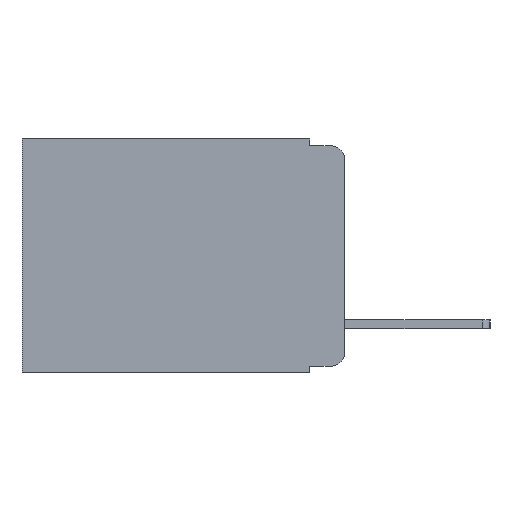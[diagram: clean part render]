
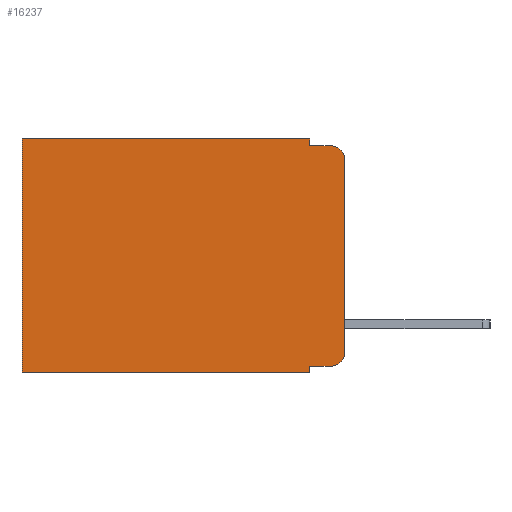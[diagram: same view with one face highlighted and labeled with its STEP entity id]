
A CAD part, left-side view. The second image highlights one B-rep face of the part: STEP entity #16237.
In plain terms, the highlighted planar face has unit normal (-1, 0, 0).
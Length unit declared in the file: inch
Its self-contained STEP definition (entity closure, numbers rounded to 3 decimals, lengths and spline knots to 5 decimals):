
#30 = ORIENTED_EDGE ( 'NONE', *, *, #7770, .T. ) ;
#162 = DIRECTION ( 'NONE',  ( 0., 0., -1. ) ) ;
#414 = ORIENTED_EDGE ( 'NONE', *, *, #9971, .T. ) ;
#877 = VERTEX_POINT ( 'NONE', #4675 ) ;
#891 = CARTESIAN_POINT ( 'NONE',  ( 0.298, 0.051, 0. ) ) ;
#1987 = CARTESIAN_POINT ( 'NONE',  ( 0.298, 0.02, -0.01 ) ) ;
#2524 = VECTOR ( 'NONE', #8147, 39.37008 ) ;
#2715 = VERTEX_POINT ( 'NONE', #1987 ) ;
#3060 = VECTOR ( 'NONE', #19576, 39.37008 ) ;
#3420 = AXIS2_PLACEMENT_3D ( 'NONE', #16864, #5910, #18692 ) ;
#3808 = EDGE_CURVE ( 'NONE', #14345, #7878, #23529, .T. ) ;
#4283 = CARTESIAN_POINT ( 'NONE',  ( 0.298, 0.473, -0.343 ) ) ;
#4372 = CARTESIAN_POINT ( 'NONE',  ( 0.298, 0.02, -0.313 ) ) ;
#4472 = EDGE_CURVE ( 'NONE', #6356, #877, #17974, .T. ) ;
#4675 = CARTESIAN_POINT ( 'NONE',  ( 0.298, 0.051, -0.01 ) ) ;
#5412 = VERTEX_POINT ( 'NONE', #4283 ) ;
#5910 = DIRECTION ( 'NONE',  ( -1., 0., 0. ) ) ;
#6225 = VECTOR ( 'NONE', #12115, 39.37008 ) ;
#6262 = CARTESIAN_POINT ( 'NONE',  ( 0.298, 0., -0.313 ) ) ;
#6305 = DIRECTION ( 'NONE',  ( 0., 0., -1. ) ) ;
#6356 = VERTEX_POINT ( 'NONE', #14288 ) ;
#6496 = VERTEX_POINT ( 'NONE', #21785 ) ;
#7347 = VECTOR ( 'NONE', #19860, 39.37008 ) ;
#7444 = ORIENTED_EDGE ( 'NONE', *, *, #21544, .F. ) ;
#7580 = LINE ( 'NONE', #13575, #2524 ) ;
#7753 = PLANE ( 'NONE',  #16686 ) ;
#7770 = EDGE_CURVE ( 'NONE', #14345, #2715, #19234, .T. ) ;
#7878 = VERTEX_POINT ( 'NONE', #6262 ) ;
#8122 = ORIENTED_EDGE ( 'NONE', *, *, #12481, .T. ) ;
#8147 = DIRECTION ( 'NONE',  ( 0., -1., 0. ) ) ;
#8908 = VECTOR ( 'NONE', #19803, 39.37008 ) ;
#9217 = VECTOR ( 'NONE', #9309, 39.37008 ) ;
#9309 = DIRECTION ( 'NONE',  ( 0., 0., -1. ) ) ;
#9953 = CARTESIAN_POINT ( 'NONE',  ( 0.298, 0.051, -0.01 ) ) ;
#9971 = EDGE_CURVE ( 'NONE', #12214, #7878, #18756, .T. ) ;
#10172 = AXIS2_PLACEMENT_3D ( 'NONE', #4372, #17206, #6305 ) ;
#10758 = ORIENTED_EDGE ( 'NONE', *, *, #3808, .F. ) ;
#11193 = DIRECTION ( 'NONE',  ( 0., 0., -1. ) ) ;
#11417 = DIRECTION ( 'NONE',  ( 1., 0., 0. ) ) ;
#11802 = DIRECTION ( 'NONE',  ( 0., -1., 0. ) ) ;
#12115 = DIRECTION ( 'NONE',  ( 0., 0., -1. ) ) ;
#12214 = VERTEX_POINT ( 'NONE', #21737 ) ;
#12231 = FACE_OUTER_BOUND ( 'NONE', #12458, .T. ) ;
#12458 = EDGE_LOOP ( 'NONE', ( #10758, #30, #15771, #22301, #12653, #18319, #7444, #18349, #8122, #414 ) ) ;
#12481 = EDGE_CURVE ( 'NONE', #18225, #12214, #7580, .T. ) ;
#12653 = ORIENTED_EDGE ( 'NONE', *, *, #16682, .T. ) ;
#13575 = CARTESIAN_POINT ( 'NONE',  ( 0.298, 0.051, -0.333 ) ) ;
#14161 = CARTESIAN_POINT ( 'NONE',  ( 0.298, 0., -0.343 ) ) ;
#14288 = CARTESIAN_POINT ( 'NONE',  ( 0.298, 0.051, 0. ) ) ;
#14345 = VERTEX_POINT ( 'NONE', #15880 ) ;
#14607 = EDGE_CURVE ( 'NONE', #6496, #5412, #22913, .T. ) ;
#14726 = CARTESIAN_POINT ( 'NONE',  ( 0.298, 0., 0. ) ) ;
#15369 = CARTESIAN_POINT ( 'NONE',  ( 0.298, 0.051, -0.333 ) ) ;
#15426 = EDGE_CURVE ( 'NONE', #18225, #16553, #20183, .T. ) ;
#15526 = VECTOR ( 'NONE', #11802, 39.37008 ) ;
#15771 = ORIENTED_EDGE ( 'NONE', *, *, #18252, .F. ) ;
#15880 = CARTESIAN_POINT ( 'NONE',  ( 0.298, 0., -0.03 ) ) ;
#16237 = ADVANCED_FACE ( 'NONE', ( #12231 ), #7753, .F. ) ;
#16553 = VERTEX_POINT ( 'NONE', #17736 ) ;
#16682 = EDGE_CURVE ( 'NONE', #6356, #6496, #22306, .T. ) ;
#16686 = AXIS2_PLACEMENT_3D ( 'NONE', #22183, #11417, #162 ) ;
#16864 = CARTESIAN_POINT ( 'NONE',  ( 0.298, 0.02, -0.03 ) ) ;
#17206 = DIRECTION ( 'NONE',  ( -1., 0., 0. ) ) ;
#17736 = CARTESIAN_POINT ( 'NONE',  ( 0.298, 0.051, -0.343 ) ) ;
#17974 = LINE ( 'NONE', #18062, #8908 ) ;
#18062 = CARTESIAN_POINT ( 'NONE',  ( 0.298, 0.051, 0. ) ) ;
#18126 = CARTESIAN_POINT ( 'NONE',  ( 0.298, 0., 0. ) ) ;
#18225 = VERTEX_POINT ( 'NONE', #15369 ) ;
#18252 = EDGE_CURVE ( 'NONE', #877, #2715, #20328, .T. ) ;
#18319 = ORIENTED_EDGE ( 'NONE', *, *, #14607, .T. ) ;
#18349 = ORIENTED_EDGE ( 'NONE', *, *, #15426, .F. ) ;
#18692 = DIRECTION ( 'NONE',  ( 0., 0., -1. ) ) ;
#18756 = CIRCLE ( 'NONE', #10172, 0.02 ) ;
#18762 = VECTOR ( 'NONE', #11193, 39.37008 ) ;
#19234 = CIRCLE ( 'NONE', #3420, 0.02 ) ;
#19576 = DIRECTION ( 'NONE',  ( 0., 1., 0. ) ) ;
#19803 = DIRECTION ( 'NONE',  ( 0., 0., -1. ) ) ;
#19860 = DIRECTION ( 'NONE',  ( 0., 1., 0. ) ) ;
#20183 = LINE ( 'NONE', #891, #6225 ) ;
#20328 = LINE ( 'NONE', #9953, #15526 ) ;
#21544 = EDGE_CURVE ( 'NONE', #16553, #5412, #22447, .T. ) ;
#21737 = CARTESIAN_POINT ( 'NONE',  ( 0.298, 0.02, -0.333 ) ) ;
#21785 = CARTESIAN_POINT ( 'NONE',  ( 0.298, 0.473, 0. ) ) ;
#21965 = CARTESIAN_POINT ( 'NONE',  ( 0.298, 0.473, 0. ) ) ;
#22183 = CARTESIAN_POINT ( 'NONE',  ( 0.298, 0., 0. ) ) ;
#22301 = ORIENTED_EDGE ( 'NONE', *, *, #4472, .F. ) ;
#22306 = LINE ( 'NONE', #18126, #7347 ) ;
#22447 = LINE ( 'NONE', #14161, #3060 ) ;
#22913 = LINE ( 'NONE', #21965, #18762 ) ;
#23529 = LINE ( 'NONE', #14726, #9217 ) ;
